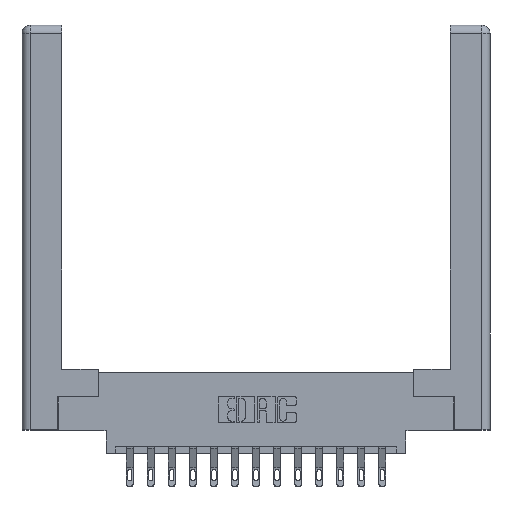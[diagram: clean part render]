
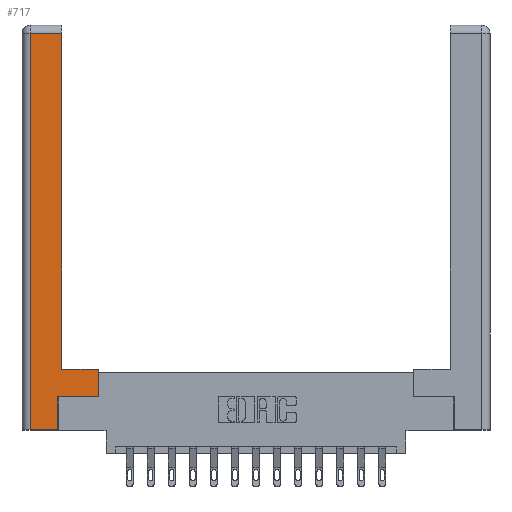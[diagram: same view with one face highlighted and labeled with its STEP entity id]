
A CAD part, top view. The second image highlights one B-rep face of the part: STEP entity #717.
In plain terms, the highlighted planar face has unit normal (0, 0, 1).
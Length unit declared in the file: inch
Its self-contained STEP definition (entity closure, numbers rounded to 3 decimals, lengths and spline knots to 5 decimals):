
#255 = EDGE_CURVE ( 'NONE', #4848, #8198, #12687, .T. ) ;
#458 = CARTESIAN_POINT ( 'NONE',  ( 0.265, 0., 0. ) ) ;
#600 = VERTEX_POINT ( 'NONE', #4948 ) ;
#615 = ORIENTED_EDGE ( 'NONE', *, *, #6775, .T. ) ;
#624 = DIRECTION ( 'NONE',  ( -1., 0., 0. ) ) ;
#717 = ADVANCED_FACE ( 'NONE', ( #15131 ), #4304, .F. ) ;
#775 = DIRECTION ( 'NONE',  ( 0., 1., 0. ) ) ;
#1441 = DIRECTION ( 'NONE',  ( 0., 1., 0. ) ) ;
#1501 = VERTEX_POINT ( 'NONE', #3515 ) ;
#1588 = ORIENTED_EDGE ( 'NONE', *, *, #3049, .T. ) ;
#1689 = AXIS2_PLACEMENT_3D ( 'NONE', #5594, #4467, #624 ) ;
#2312 = LINE ( 'NONE', #7107, #16425 ) ;
#2320 = DIRECTION ( 'NONE',  ( -1., 0., 0. ) ) ;
#2354 = EDGE_CURVE ( 'NONE', #1501, #15914, #15570, .T. ) ;
#2693 = CARTESIAN_POINT ( 'NONE',  ( 0.0615, 2.94, 0. ) ) ;
#2703 = LINE ( 'NONE', #6641, #14396 ) ;
#3049 = EDGE_CURVE ( 'NONE', #5515, #10598, #14750, .T. ) ;
#3515 = CARTESIAN_POINT ( 'NONE',  ( 0.295, 2.94, 0. ) ) ;
#3546 = CARTESIAN_POINT ( 'NONE',  ( 0.565, 0.45, 0. ) ) ;
#3773 = CARTESIAN_POINT ( 'NONE',  ( 0.565, 0.45, 0. ) ) ;
#4065 = EDGE_LOOP ( 'NONE', ( #12209, #12463, #615, #7389, #10062, #6316, #1588, #5672 ) ) ;
#4304 = PLANE ( 'NONE',  #1689 ) ;
#4467 = DIRECTION ( 'NONE',  ( 0., 0., -1. ) ) ;
#4542 = CARTESIAN_POINT ( 'NONE',  ( 0.265, 0., 0. ) ) ;
#4848 = VERTEX_POINT ( 'NONE', #15251 ) ;
#4903 = CARTESIAN_POINT ( 'NONE',  ( 0.295, 0.45, 0. ) ) ;
#4948 = CARTESIAN_POINT ( 'NONE',  ( 0.265, 0.245, 0. ) ) ;
#5510 = DIRECTION ( 'NONE',  ( 0., 1., 0. ) ) ;
#5515 = VERTEX_POINT ( 'NONE', #6194 ) ;
#5594 = CARTESIAN_POINT ( 'NONE',  ( 0., 0., 0. ) ) ;
#5672 = ORIENTED_EDGE ( 'NONE', *, *, #16562, .T. ) ;
#5749 = VECTOR ( 'NONE', #13744, 39.37008 ) ;
#6008 = VECTOR ( 'NONE', #2320, 39.37008 ) ;
#6194 = CARTESIAN_POINT ( 'NONE',  ( 0.565, 0.245, 0. ) ) ;
#6316 = ORIENTED_EDGE ( 'NONE', *, *, #16336, .T. ) ;
#6537 = VECTOR ( 'NONE', #5510, 39.37008 ) ;
#6641 = CARTESIAN_POINT ( 'NONE',  ( 0.295, 3., 0. ) ) ;
#6775 = EDGE_CURVE ( 'NONE', #15914, #4848, #12740, .T. ) ;
#7107 = CARTESIAN_POINT ( 'NONE',  ( 0.265, 0.245, 0. ) ) ;
#7389 = ORIENTED_EDGE ( 'NONE', *, *, #255, .T. ) ;
#8020 = LINE ( 'NONE', #10651, #12307 ) ;
#8198 = VERTEX_POINT ( 'NONE', #458 ) ;
#10062 = ORIENTED_EDGE ( 'NONE', *, *, #10466, .T. ) ;
#10466 = EDGE_CURVE ( 'NONE', #8198, #600, #2312, .T. ) ;
#10598 = VERTEX_POINT ( 'NONE', #3546 ) ;
#10651 = CARTESIAN_POINT ( 'NONE',  ( 0.565, 0.245, 0. ) ) ;
#10686 = LINE ( 'NONE', #12598, #6008 ) ;
#10895 = DIRECTION ( 'NONE',  ( 1., 0., 0. ) ) ;
#11320 = CARTESIAN_POINT ( 'NONE',  ( 0.0615, 0., 0. ) ) ;
#12113 = VECTOR ( 'NONE', #12520, 39.37008 ) ;
#12209 = ORIENTED_EDGE ( 'NONE', *, *, #16134, .T. ) ;
#12307 = VECTOR ( 'NONE', #10895, 39.37008 ) ;
#12463 = ORIENTED_EDGE ( 'NONE', *, *, #2354, .T. ) ;
#12520 = DIRECTION ( 'NONE',  ( 0., -1., 0. ) ) ;
#12598 = CARTESIAN_POINT ( 'NONE',  ( 0.295, 0.45, 0. ) ) ;
#12687 = LINE ( 'NONE', #4542, #5749 ) ;
#12740 = LINE ( 'NONE', #11320, #12113 ) ;
#12845 = VERTEX_POINT ( 'NONE', #4903 ) ;
#13744 = DIRECTION ( 'NONE',  ( 1., 0., 0. ) ) ;
#14396 = VECTOR ( 'NONE', #1441, 39.37008 ) ;
#14750 = LINE ( 'NONE', #3773, #6537 ) ;
#15131 = FACE_OUTER_BOUND ( 'NONE', #4065, .T. ) ;
#15251 = CARTESIAN_POINT ( 'NONE',  ( 0.0615, 0., 0. ) ) ;
#15375 = VECTOR ( 'NONE', #15796, 39.37008 ) ;
#15570 = LINE ( 'NONE', #2693, #15375 ) ;
#15796 = DIRECTION ( 'NONE',  ( -1., 0., 0. ) ) ;
#15914 = VERTEX_POINT ( 'NONE', #16551 ) ;
#16134 = EDGE_CURVE ( 'NONE', #12845, #1501, #2703, .T. ) ;
#16336 = EDGE_CURVE ( 'NONE', #600, #5515, #8020, .T. ) ;
#16425 = VECTOR ( 'NONE', #775, 39.37008 ) ;
#16551 = CARTESIAN_POINT ( 'NONE',  ( 0.0615, 2.94, 0. ) ) ;
#16562 = EDGE_CURVE ( 'NONE', #10598, #12845, #10686, .T. ) ;
